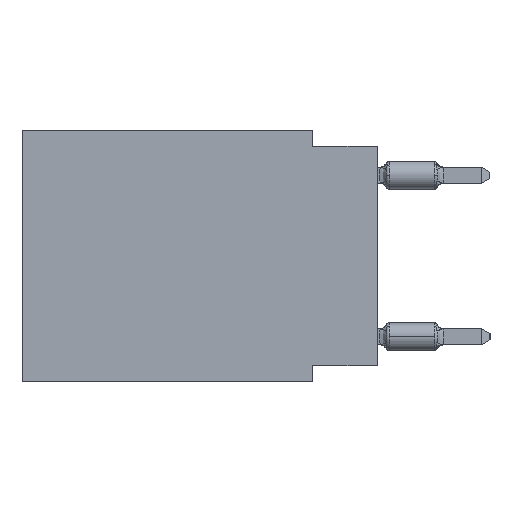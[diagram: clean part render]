
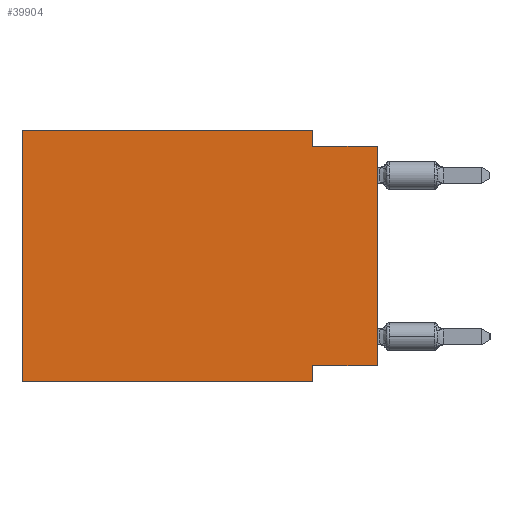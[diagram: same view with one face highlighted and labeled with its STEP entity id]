
A CAD part, left-side view. The second image highlights one B-rep face of the part: STEP entity #39904.
In plain terms, the highlighted planar face has unit normal (-1, 0, 0).
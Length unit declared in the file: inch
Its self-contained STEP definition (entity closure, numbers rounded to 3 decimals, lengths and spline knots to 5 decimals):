
#2793 = CARTESIAN_POINT ( 'NONE',  ( 0., 0.55, 0. ) ) ;
#3054 = CARTESIAN_POINT ( 'NONE',  ( 0., 0.55, 0. ) ) ;
#3066 = ORIENTED_EDGE ( 'NONE', *, *, #9199, .T. ) ;
#3150 = LINE ( 'NONE', #33634, #37490 ) ;
#3316 = VERTEX_POINT ( 'NONE', #49379 ) ;
#4772 = VECTOR ( 'NONE', #26346, 39.37008 ) ;
#5166 = VERTEX_POINT ( 'NONE', #21686 ) ;
#5221 = VECTOR ( 'NONE', #44755, 39.37008 ) ;
#5369 = DIRECTION ( 'NONE',  ( 0., 0., -1. ) ) ;
#7441 = DIRECTION ( 'NONE',  ( 0., 0., 1. ) ) ;
#9141 = CARTESIAN_POINT ( 'NONE',  ( 0., 0.55, 0. ) ) ;
#9199 = EDGE_CURVE ( 'NONE', #48103, #5166, #20768, .T. ) ;
#9220 = VECTOR ( 'NONE', #18050, 39.37008 ) ;
#10553 = VERTEX_POINT ( 'NONE', #21509 ) ;
#11871 = VERTEX_POINT ( 'NONE', #42552 ) ;
#12635 = FACE_OUTER_BOUND ( 'NONE', #46691, .T. ) ;
#13573 = CARTESIAN_POINT ( 'NONE',  ( 0., 0.55, -0.39 ) ) ;
#18013 = CARTESIAN_POINT ( 'NONE',  ( 0., 0.1, 0. ) ) ;
#18050 = DIRECTION ( 'NONE',  ( 0., 0., 1. ) ) ;
#18455 = EDGE_CURVE ( 'NONE', #19184, #11871, #37275, .T. ) ;
#19091 = EDGE_CURVE ( 'NONE', #10553, #19520, #3150, .T. ) ;
#19184 = VERTEX_POINT ( 'NONE', #34998 ) ;
#19520 = VERTEX_POINT ( 'NONE', #30463 ) ;
#20097 = AXIS2_PLACEMENT_3D ( 'NONE', #9141, #39602, #5369 ) ;
#20277 = DIRECTION ( 'NONE',  ( 0., -1., 0. ) ) ;
#20768 = LINE ( 'NONE', #43016, #29113 ) ;
#21509 = CARTESIAN_POINT ( 'NONE',  ( 0., 0., -0.365 ) ) ;
#21686 = CARTESIAN_POINT ( 'NONE',  ( 0., 0.1, -0.39 ) ) ;
#22748 = ORIENTED_EDGE ( 'NONE', *, *, #28699, .T. ) ;
#24492 = ORIENTED_EDGE ( 'NONE', *, *, #19091, .F. ) ;
#24629 = EDGE_CURVE ( 'NONE', #11871, #3316, #29259, .T. ) ;
#26346 = DIRECTION ( 'NONE',  ( 0., 0., -1. ) ) ;
#27864 = PLANE ( 'NONE',  #20097 ) ;
#28301 = CARTESIAN_POINT ( 'NONE',  ( 0., 0., -0.025 ) ) ;
#28699 = EDGE_CURVE ( 'NONE', #10553, #36780, #33412, .T. ) ;
#29113 = VECTOR ( 'NONE', #20277, 39.37008 ) ;
#29259 = LINE ( 'NONE', #18013, #5221 ) ;
#29361 = LINE ( 'NONE', #33116, #4772 ) ;
#30463 = CARTESIAN_POINT ( 'NONE',  ( 0., 0.1, -0.365 ) ) ;
#30726 = ORIENTED_EDGE ( 'NONE', *, *, #46373, .F. ) ;
#30926 = VECTOR ( 'NONE', #7441, 39.37008 ) ;
#33000 = ORIENTED_EDGE ( 'NONE', *, *, #24629, .F. ) ;
#33079 = EDGE_CURVE ( 'NONE', #19520, #5166, #29361, .T. ) ;
#33116 = CARTESIAN_POINT ( 'NONE',  ( 0., 0.1, -0.39 ) ) ;
#33412 = LINE ( 'NONE', #40916, #30926 ) ;
#33544 = DIRECTION ( 'NONE',  ( 0., -1., 0. ) ) ;
#33634 = CARTESIAN_POINT ( 'NONE',  ( 0., 0., -0.365 ) ) ;
#34008 = ORIENTED_EDGE ( 'NONE', *, *, #18455, .F. ) ;
#34998 = CARTESIAN_POINT ( 'NONE',  ( 0., 0.55, 0. ) ) ;
#36113 = EDGE_CURVE ( 'NONE', #3316, #36780, #37423, .T. ) ;
#36780 = VERTEX_POINT ( 'NONE', #39129 ) ;
#37013 = LINE ( 'NONE', #2793, #9220 ) ;
#37275 = LINE ( 'NONE', #3054, #46267 ) ;
#37423 = LINE ( 'NONE', #28301, #41483 ) ;
#37490 = VECTOR ( 'NONE', #48888, 39.37008 ) ;
#39129 = CARTESIAN_POINT ( 'NONE',  ( 0., 0., -0.025 ) ) ;
#39602 = DIRECTION ( 'NONE',  ( 1., 0., 0. ) ) ;
#39795 = ORIENTED_EDGE ( 'NONE', *, *, #36113, .F. ) ;
#39904 = ADVANCED_FACE ( 'NONE', ( #12635 ), #27864, .F. ) ;
#40916 = CARTESIAN_POINT ( 'NONE',  ( 0., 0., 0. ) ) ;
#41434 = DIRECTION ( 'NONE',  ( 0., -1., 0. ) ) ;
#41483 = VECTOR ( 'NONE', #41434, 39.37008 ) ;
#42552 = CARTESIAN_POINT ( 'NONE',  ( 0., 0.1, 0. ) ) ;
#43016 = CARTESIAN_POINT ( 'NONE',  ( 0., 0.55, -0.39 ) ) ;
#44755 = DIRECTION ( 'NONE',  ( 0., 0., -1. ) ) ;
#46267 = VECTOR ( 'NONE', #33544, 39.37008 ) ;
#46373 = EDGE_CURVE ( 'NONE', #48103, #19184, #37013, .T. ) ;
#46691 = EDGE_LOOP ( 'NONE', ( #22748, #39795, #33000, #34008, #30726, #3066, #47059, #24492 ) ) ;
#47059 = ORIENTED_EDGE ( 'NONE', *, *, #33079, .F. ) ;
#48103 = VERTEX_POINT ( 'NONE', #13573 ) ;
#48888 = DIRECTION ( 'NONE',  ( 0., 1., 0. ) ) ;
#49379 = CARTESIAN_POINT ( 'NONE',  ( 0., 0.1, -0.025 ) ) ;
